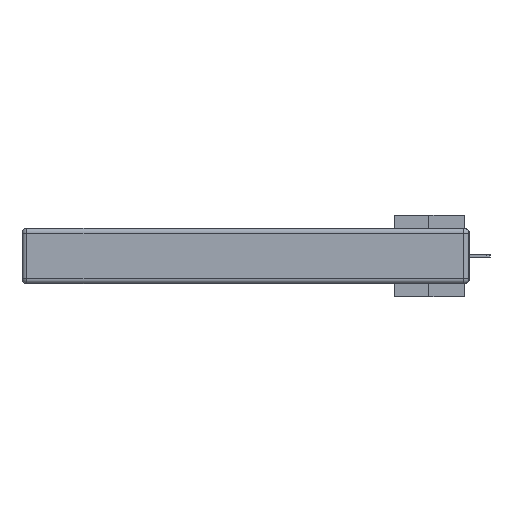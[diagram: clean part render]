
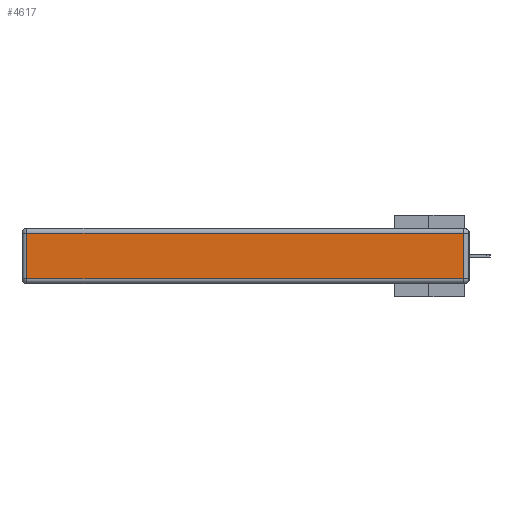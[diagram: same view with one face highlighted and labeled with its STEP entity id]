
A CAD part, left-side view. The second image highlights one B-rep face of the part: STEP entity #4617.
In plain terms, the highlighted planar face has unit normal (-1, 0, 0).
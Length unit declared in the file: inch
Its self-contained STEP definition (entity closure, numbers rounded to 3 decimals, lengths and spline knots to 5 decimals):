
#1766 = PLANE ( 'NONE',  #29645 ) ;
#2414 = ORIENTED_EDGE ( 'NONE', *, *, #16283, .T. ) ;
#3311 = CARTESIAN_POINT ( 'NONE',  ( 0., 0.03, -0.343 ) ) ;
#3701 = DIRECTION ( 'NONE',  ( 0., 0., -1. ) ) ;
#4617 = ADVANCED_FACE ( 'NONE', ( #19555 ), #1766, .T. ) ;
#6137 = CARTESIAN_POINT ( 'NONE',  ( 0., 2.72, -0.313 ) ) ;
#8140 = CARTESIAN_POINT ( 'NONE',  ( 0., 0.03, -0.03 ) ) ;
#9170 = VERTEX_POINT ( 'NONE', #32738 ) ;
#13643 = ORIENTED_EDGE ( 'NONE', *, *, #13974, .T. ) ;
#13974 = EDGE_CURVE ( 'NONE', #9170, #18070, #27006, .T. ) ;
#14208 = EDGE_CURVE ( 'NONE', #18070, #26829, #20298, .T. ) ;
#16053 = DIRECTION ( 'NONE',  ( -1., 0., 0. ) ) ;
#16207 = CARTESIAN_POINT ( 'NONE',  ( 0., 2.72, -0.343 ) ) ;
#16283 = EDGE_CURVE ( 'NONE', #26829, #20326, #21717, .T. ) ;
#17624 = CARTESIAN_POINT ( 'NONE',  ( 0., 2.72, -0.03 ) ) ;
#17873 = ORIENTED_EDGE ( 'NONE', *, *, #14208, .T. ) ;
#18070 = VERTEX_POINT ( 'NONE', #8140 ) ;
#18579 = ORIENTED_EDGE ( 'NONE', *, *, #33825, .T. ) ;
#19555 = FACE_OUTER_BOUND ( 'NONE', #37494, .T. ) ;
#20291 = VECTOR ( 'NONE', #29204, 39.37008 ) ;
#20298 = LINE ( 'NONE', #23636, #22687 ) ;
#20326 = VERTEX_POINT ( 'NONE', #6137 ) ;
#20547 = CARTESIAN_POINT ( 'NONE',  ( 0., 0., -0.313 ) ) ;
#21717 = LINE ( 'NONE', #16207, #27062 ) ;
#22687 = VECTOR ( 'NONE', #31863, 39.37008 ) ;
#23636 = CARTESIAN_POINT ( 'NONE',  ( 0., 2.75, -0.03 ) ) ;
#26829 = VERTEX_POINT ( 'NONE', #17624 ) ;
#27006 = LINE ( 'NONE', #3311, #38324 ) ;
#27062 = VECTOR ( 'NONE', #3701, 39.37008 ) ;
#29204 = DIRECTION ( 'NONE',  ( 0., -1., 0. ) ) ;
#29645 = AXIS2_PLACEMENT_3D ( 'NONE', #34264, #16053, #30950 ) ;
#30950 = DIRECTION ( 'NONE',  ( 0., 0., 1. ) ) ;
#31863 = DIRECTION ( 'NONE',  ( 0., 1., 0. ) ) ;
#32507 = LINE ( 'NONE', #20547, #20291 ) ;
#32738 = CARTESIAN_POINT ( 'NONE',  ( 0., 0.03, -0.313 ) ) ;
#33825 = EDGE_CURVE ( 'NONE', #20326, #9170, #32507, .T. ) ;
#33832 = DIRECTION ( 'NONE',  ( 0., 0., 1. ) ) ;
#34264 = CARTESIAN_POINT ( 'NONE',  ( 0., 0., -0.343 ) ) ;
#37494 = EDGE_LOOP ( 'NONE', ( #18579, #13643, #17873, #2414 ) ) ;
#38324 = VECTOR ( 'NONE', #33832, 39.37008 ) ;
